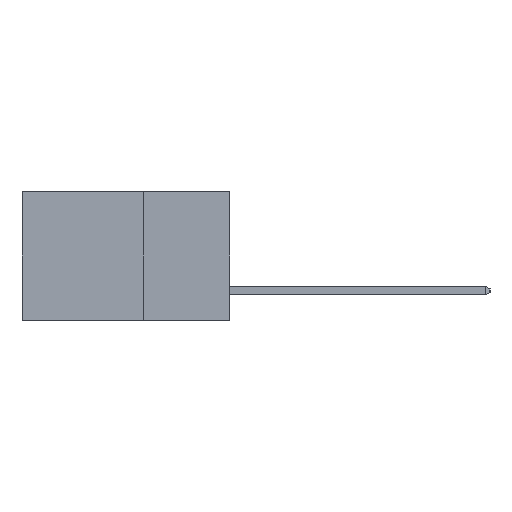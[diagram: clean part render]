
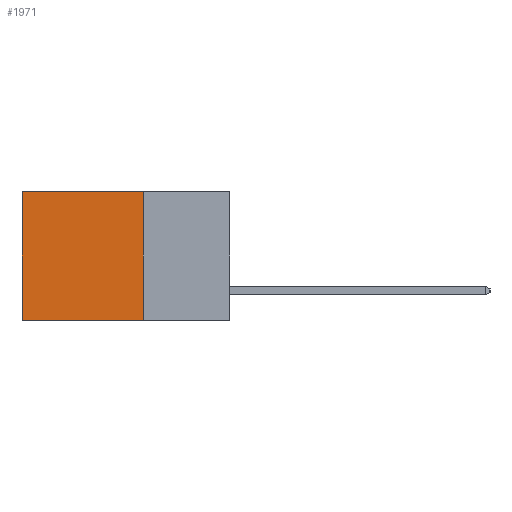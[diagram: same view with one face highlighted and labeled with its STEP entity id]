
A CAD part, left-side view. The second image highlights one B-rep face of the part: STEP entity #1971.
In plain terms, the highlighted planar face has unit normal (-1, 0, 0).
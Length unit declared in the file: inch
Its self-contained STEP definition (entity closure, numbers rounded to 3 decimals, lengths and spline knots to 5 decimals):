
#273 = PLANE ( 'NONE',  #6726 ) ;
#489 = VERTEX_POINT ( 'NONE', #13849 ) ;
#1255 = EDGE_LOOP ( 'NONE', ( #10645, #2341, #10979, #2682 ) ) ;
#1576 = EDGE_CURVE ( 'NONE', #11279, #2980, #6979, .T. ) ;
#1948 = VECTOR ( 'NONE', #6570, 39.37008 ) ;
#1971 = ADVANCED_FACE ( 'NONE', ( #4774 ), #273, .F. ) ;
#2003 = CARTESIAN_POINT ( 'NONE',  ( 0.298, 0.25, 0. ) ) ;
#2341 = ORIENTED_EDGE ( 'NONE', *, *, #8377, .F. ) ;
#2682 = ORIENTED_EDGE ( 'NONE', *, *, #13455, .T. ) ;
#2980 = VERTEX_POINT ( 'NONE', #7311 ) ;
#3424 = CARTESIAN_POINT ( 'NONE',  ( 0.298, 0.25, 0. ) ) ;
#3754 = VERTEX_POINT ( 'NONE', #12220 ) ;
#4217 = CARTESIAN_POINT ( 'NONE',  ( 0.298, 0.25, 0. ) ) ;
#4250 = VECTOR ( 'NONE', #10786, 39.37008 ) ;
#4731 = EDGE_CURVE ( 'NONE', #3754, #489, #8070, .T. ) ;
#4774 = FACE_OUTER_BOUND ( 'NONE', #1255, .T. ) ;
#5361 = CARTESIAN_POINT ( 'NONE',  ( 0.298, 0.25, -0.37 ) ) ;
#5390 = DIRECTION ( 'NONE',  ( 0., 0., -1. ) ) ;
#6570 = DIRECTION ( 'NONE',  ( 0., 0., -1. ) ) ;
#6638 = VECTOR ( 'NONE', #5390, 39.37008 ) ;
#6726 = AXIS2_PLACEMENT_3D ( 'NONE', #9087, #6937, #6907 ) ;
#6907 = DIRECTION ( 'NONE',  ( 0., 0., -1. ) ) ;
#6937 = DIRECTION ( 'NONE',  ( 1., 0., 0. ) ) ;
#6979 = LINE ( 'NONE', #2003, #6638 ) ;
#7100 = LINE ( 'NONE', #5361, #4250 ) ;
#7311 = CARTESIAN_POINT ( 'NONE',  ( 0.298, 0.25, -0.37 ) ) ;
#8070 = LINE ( 'NONE', #10756, #1948 ) ;
#8377 = EDGE_CURVE ( 'NONE', #2980, #489, #7100, .T. ) ;
#9087 = CARTESIAN_POINT ( 'NONE',  ( 0.298, 0.25, 0. ) ) ;
#10645 = ORIENTED_EDGE ( 'NONE', *, *, #4731, .T. ) ;
#10756 = CARTESIAN_POINT ( 'NONE',  ( 0.298, 0.6, 0. ) ) ;
#10786 = DIRECTION ( 'NONE',  ( 0., 1., 0. ) ) ;
#10979 = ORIENTED_EDGE ( 'NONE', *, *, #1576, .F. ) ;
#11088 = VECTOR ( 'NONE', #12036, 39.37008 ) ;
#11279 = VERTEX_POINT ( 'NONE', #4217 ) ;
#12036 = DIRECTION ( 'NONE',  ( 0., 1., 0. ) ) ;
#12220 = CARTESIAN_POINT ( 'NONE',  ( 0.298, 0.6, 0. ) ) ;
#13455 = EDGE_CURVE ( 'NONE', #11279, #3754, #13790, .T. ) ;
#13790 = LINE ( 'NONE', #3424, #11088 ) ;
#13849 = CARTESIAN_POINT ( 'NONE',  ( 0.298, 0.6, -0.37 ) ) ;
